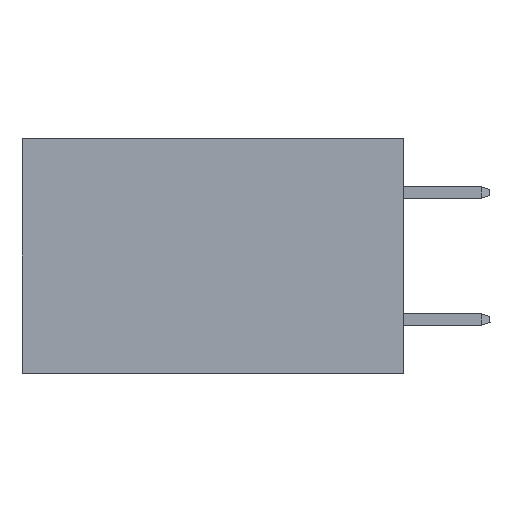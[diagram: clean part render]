
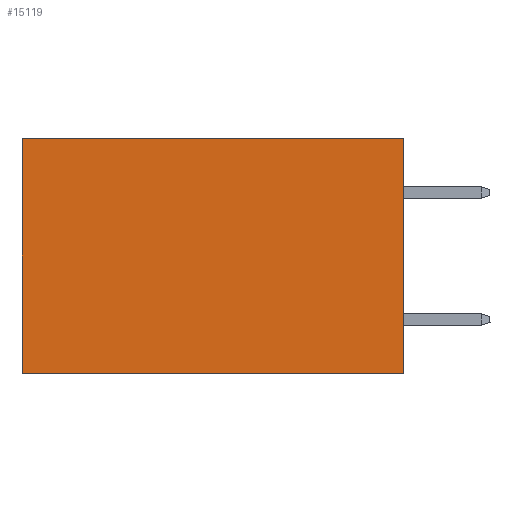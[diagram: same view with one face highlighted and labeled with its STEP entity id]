
A CAD part, left-side view. The second image highlights one B-rep face of the part: STEP entity #15119.
In plain terms, the highlighted planar face has unit normal (-1, 0, 0).
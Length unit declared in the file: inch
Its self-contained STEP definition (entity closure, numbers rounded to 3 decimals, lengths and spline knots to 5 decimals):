
#559 = CARTESIAN_POINT ( 'NONE',  ( 0.2875, 0., -0.37 ) ) ;
#1607 = DIRECTION ( 'NONE',  ( 0., 0., -1. ) ) ;
#1789 = VERTEX_POINT ( 'NONE', #9750 ) ;
#2759 = EDGE_CURVE ( 'NONE', #3005, #19734, #11140, .T. ) ;
#3005 = VERTEX_POINT ( 'NONE', #15278 ) ;
#4153 = VECTOR ( 'NONE', #15451, 39.37008 ) ;
#4315 = ORIENTED_EDGE ( 'NONE', *, *, #8089, .T. ) ;
#4378 = EDGE_CURVE ( 'NONE', #19734, #18086, #17845, .T. ) ;
#4442 = AXIS2_PLACEMENT_3D ( 'NONE', #24382, #10924, #1607 ) ;
#5115 = CARTESIAN_POINT ( 'NONE',  ( 0.2875, 0., 0. ) ) ;
#5259 = VECTOR ( 'NONE', #6324, 39.37008 ) ;
#6324 = DIRECTION ( 'NONE',  ( 0., 1., 0. ) ) ;
#6446 = CARTESIAN_POINT ( 'NONE',  ( 0.2875, 0., -0.37 ) ) ;
#8089 = EDGE_CURVE ( 'NONE', #1789, #18086, #20359, .T. ) ;
#8786 = CARTESIAN_POINT ( 'NONE',  ( 0.2875, 0.6, 0. ) ) ;
#9750 = CARTESIAN_POINT ( 'NONE',  ( 0.2875, 0.6, 0. ) ) ;
#10172 = VECTOR ( 'NONE', #16521, 39.37008 ) ;
#10425 = CARTESIAN_POINT ( 'NONE',  ( 0.2875, 0., 0. ) ) ;
#10794 = LINE ( 'NONE', #5115, #4153 ) ;
#10924 = DIRECTION ( 'NONE',  ( 1., 0., 0. ) ) ;
#11140 = LINE ( 'NONE', #10425, #22621 ) ;
#13183 = CARTESIAN_POINT ( 'NONE',  ( 0.2875, 0.6, -0.37 ) ) ;
#13836 = EDGE_CURVE ( 'NONE', #3005, #1789, #10794, .T. ) ;
#14337 = ORIENTED_EDGE ( 'NONE', *, *, #2759, .F. ) ;
#15119 = ADVANCED_FACE ( 'NONE', ( #17125 ), #19048, .F. ) ;
#15278 = CARTESIAN_POINT ( 'NONE',  ( 0.2875, 0., 0. ) ) ;
#15451 = DIRECTION ( 'NONE',  ( 0., 1., 0. ) ) ;
#16499 = DIRECTION ( 'NONE',  ( 0., 0., -1. ) ) ;
#16521 = DIRECTION ( 'NONE',  ( 0., 0., -1. ) ) ;
#17125 = FACE_OUTER_BOUND ( 'NONE', #18129, .T. ) ;
#17845 = LINE ( 'NONE', #559, #5259 ) ;
#18086 = VERTEX_POINT ( 'NONE', #13183 ) ;
#18129 = EDGE_LOOP ( 'NONE', ( #4315, #20997, #14337, #24110 ) ) ;
#19048 = PLANE ( 'NONE',  #4442 ) ;
#19734 = VERTEX_POINT ( 'NONE', #6446 ) ;
#20359 = LINE ( 'NONE', #8786, #10172 ) ;
#20997 = ORIENTED_EDGE ( 'NONE', *, *, #4378, .F. ) ;
#22621 = VECTOR ( 'NONE', #16499, 39.37008 ) ;
#24110 = ORIENTED_EDGE ( 'NONE', *, *, #13836, .T. ) ;
#24382 = CARTESIAN_POINT ( 'NONE',  ( 0.2875, 0., 0. ) ) ;
